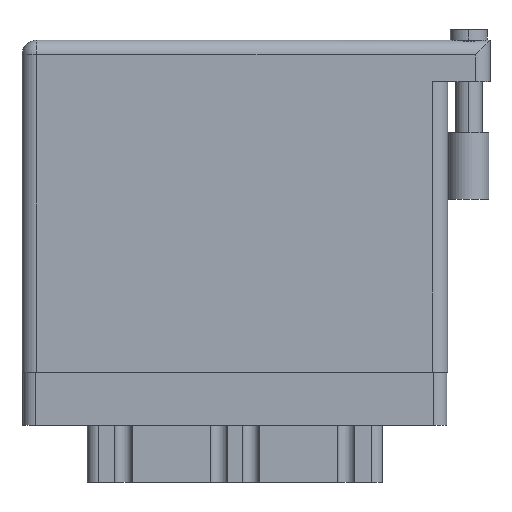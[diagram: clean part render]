
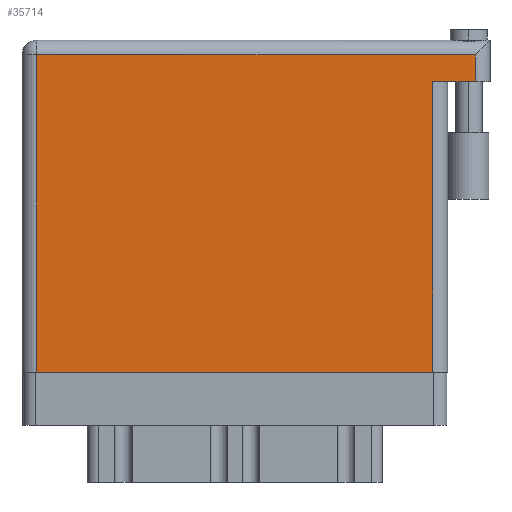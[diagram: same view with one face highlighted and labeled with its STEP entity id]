
A CAD part, front view. The second image highlights one B-rep face of the part: STEP entity #35714.
In plain terms, the highlighted face is planar.
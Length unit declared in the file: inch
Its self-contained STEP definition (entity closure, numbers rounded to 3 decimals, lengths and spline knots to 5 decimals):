
#946 = CARTESIAN_POINT ( 'NONE',  ( 0., 1.496, 0. ) ) ;
#1423 = CARTESIAN_POINT ( 'NONE',  ( 1.938, 1.369, 0. ) ) ;
#5873 = DIRECTION ( 'NONE',  ( -1., 0., 0. ) ) ;
#6100 = VECTOR ( 'NONE', #30525, 39.37008 ) ;
#6908 = LINE ( 'NONE', #28079, #35619 ) ;
#8801 = DIRECTION ( 'NONE',  ( 0., 0., -1. ) ) ;
#9349 = EDGE_CURVE ( 'NONE', #34603, #24784, #19716, .T. ) ;
#9527 = CARTESIAN_POINT ( 'NONE',  ( 0.07, 0., 0. ) ) ;
#10196 = DIRECTION ( 'NONE',  ( -1., 0., 0. ) ) ;
#10298 = ORIENTED_EDGE ( 'NONE', *, *, #26257, .T. ) ;
#11011 = CARTESIAN_POINT ( 'NONE',  ( 1.938, 1.369, 0. ) ) ;
#12594 = AXIS2_PLACEMENT_3D ( 'NONE', #37765, #8801, #5873 ) ;
#12795 = DIRECTION ( 'NONE',  ( -1., 0., 0. ) ) ;
#13275 = DIRECTION ( 'NONE',  ( 0., 1., 0. ) ) ;
#13696 = VECTOR ( 'NONE', #12795, 39.37008 ) ;
#13872 = FACE_OUTER_BOUND ( 'NONE', #30453, .T. ) ;
#14052 = CARTESIAN_POINT ( 'NONE',  ( 0.07, 0., 0. ) ) ;
#15457 = EDGE_CURVE ( 'NONE', #19521, #24784, #33677, .T. ) ;
#15726 = LINE ( 'NONE', #946, #13696 ) ;
#18116 = LINE ( 'NONE', #9527, #28830 ) ;
#18280 = ORIENTED_EDGE ( 'NONE', *, *, #28906, .T. ) ;
#19210 = ORIENTED_EDGE ( 'NONE', *, *, #32991, .T. ) ;
#19521 = VERTEX_POINT ( 'NONE', #31726 ) ;
#19716 = LINE ( 'NONE', #33718, #35355 ) ;
#21219 = CARTESIAN_POINT ( 'NONE',  ( 0., 0., 0. ) ) ;
#24224 = ORIENTED_EDGE ( 'NONE', *, *, #38342, .T. ) ;
#24784 = VERTEX_POINT ( 'NONE', #11011 ) ;
#26115 = ORIENTED_EDGE ( 'NONE', *, *, #15457, .T. ) ;
#26257 = EDGE_CURVE ( 'NONE', #35118, #35175, #18116, .T. ) ;
#27822 = CARTESIAN_POINT ( 'NONE',  ( 2.138, 1.496, 0. ) ) ;
#28079 = CARTESIAN_POINT ( 'NONE',  ( 2.138, 1.566, 0. ) ) ;
#28830 = VECTOR ( 'NONE', #36350, 39.37008 ) ;
#28906 = EDGE_CURVE ( 'NONE', #35175, #19521, #33831, .T. ) ;
#30049 = CARTESIAN_POINT ( 'NONE',  ( 2.138, 1.369, 0. ) ) ;
#30226 = VERTEX_POINT ( 'NONE', #27822 ) ;
#30434 = ORIENTED_EDGE ( 'NONE', *, *, #9349, .F. ) ;
#30453 = EDGE_LOOP ( 'NONE', ( #18280, #26115, #30434, #24224, #19210, #10298 ) ) ;
#30525 = DIRECTION ( 'NONE',  ( 1., 0., 0. ) ) ;
#31347 = CARTESIAN_POINT ( 'NONE',  ( 0.07, 1.496, 0. ) ) ;
#31726 = CARTESIAN_POINT ( 'NONE',  ( 1.938, 0., 0. ) ) ;
#32991 = EDGE_CURVE ( 'NONE', #30226, #35118, #15726, .T. ) ;
#33677 = LINE ( 'NONE', #1423, #36920 ) ;
#33718 = CARTESIAN_POINT ( 'NONE',  ( 2.208, 1.369, 0. ) ) ;
#33831 = LINE ( 'NONE', #21219, #6100 ) ;
#34603 = VERTEX_POINT ( 'NONE', #30049 ) ;
#35118 = VERTEX_POINT ( 'NONE', #31347 ) ;
#35175 = VERTEX_POINT ( 'NONE', #14052 ) ;
#35355 = VECTOR ( 'NONE', #10196, 39.37008 ) ;
#35619 = VECTOR ( 'NONE', #36658, 39.37008 ) ;
#35714 = ADVANCED_FACE ( 'NONE', ( #13872 ), #37568, .F. ) ;
#36350 = DIRECTION ( 'NONE',  ( 0., -1., 0. ) ) ;
#36658 = DIRECTION ( 'NONE',  ( 0., 1., 0. ) ) ;
#36920 = VECTOR ( 'NONE', #13275, 39.37008 ) ;
#37568 = PLANE ( 'NONE',  #12594 ) ;
#37765 = CARTESIAN_POINT ( 'NONE',  ( 0., 1.566, 0. ) ) ;
#38342 = EDGE_CURVE ( 'NONE', #34603, #30226, #6908, .T. ) ;
